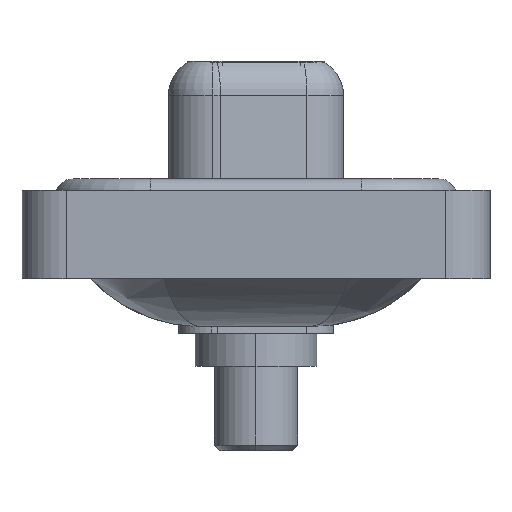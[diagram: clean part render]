
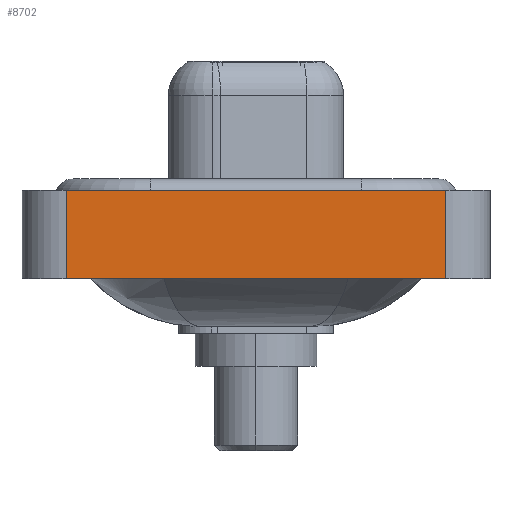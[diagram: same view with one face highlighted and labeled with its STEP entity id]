
A CAD part, left-side view. The second image highlights one B-rep face of the part: STEP entity #8702.
In plain terms, the highlighted planar face has unit normal (-1, 0, 0).
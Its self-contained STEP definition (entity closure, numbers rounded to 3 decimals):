
#165 = LINE ( 'NONE', #6627, #10528 ) ;
#203 = VECTOR ( 'NONE', #7106, 1000. ) ;
#679 = EDGE_CURVE ( 'NONE', #3708, #6044, #12628, .T. ) ;
#739 = VERTEX_POINT ( 'NONE', #1857 ) ;
#1495 = CARTESIAN_POINT ( 'NONE',  ( -7.3, 8.55, -3.6 ) ) ;
#1734 = ORIENTED_EDGE ( 'NONE', *, *, #12580, .T. ) ;
#1857 = CARTESIAN_POINT ( 'NONE',  ( -7.3, -8.55, -3.6 ) ) ;
#2555 = DIRECTION ( 'NONE',  ( 0., 0., 1. ) ) ;
#3118 = LINE ( 'NONE', #12574, #203 ) ;
#3282 = VECTOR ( 'NONE', #2555, 1000. ) ;
#3708 = VERTEX_POINT ( 'NONE', #15925 ) ;
#3989 = VECTOR ( 'NONE', #4555, 1000. ) ;
#4277 = DIRECTION ( 'NONE',  ( 0., -1., 0. ) ) ;
#4278 = CARTESIAN_POINT ( 'NONE',  ( -7.3, -8.55, 0.4 ) ) ;
#4555 = DIRECTION ( 'NONE',  ( 0., -1., 0. ) ) ;
#6044 = VERTEX_POINT ( 'NONE', #4278 ) ;
#6154 = DIRECTION ( 'NONE',  ( 0., 0., 1. ) ) ;
#6627 = CARTESIAN_POINT ( 'NONE',  ( -7.3, -8.55, -3.6 ) ) ;
#6684 = EDGE_LOOP ( 'NONE', ( #14309, #14378, #8694, #1734 ) ) ;
#7106 = DIRECTION ( 'NONE',  ( 0., 0., 1. ) ) ;
#8246 = EDGE_CURVE ( 'NONE', #739, #6044, #3118, .T. ) ;
#8694 = ORIENTED_EDGE ( 'NONE', *, *, #9217, .F. ) ;
#8702 = ADVANCED_FACE ( 'NONE', ( #9980 ), #11199, .T. ) ;
#9217 = EDGE_CURVE ( 'NONE', #12117, #3708, #14473, .T. ) ;
#9980 = FACE_OUTER_BOUND ( 'NONE', #6684, .T. ) ;
#10528 = VECTOR ( 'NONE', #4277, 1000. ) ;
#11199 = PLANE ( 'NONE',  #15180 ) ;
#12117 = VERTEX_POINT ( 'NONE', #1495 ) ;
#12506 = CARTESIAN_POINT ( 'NONE',  ( -7.3, -8.55, -3.6 ) ) ;
#12574 = CARTESIAN_POINT ( 'NONE',  ( -7.3, -8.55, -3.6 ) ) ;
#12580 = EDGE_CURVE ( 'NONE', #12117, #739, #165, .T. ) ;
#12628 = LINE ( 'NONE', #15325, #3989 ) ;
#12759 = DIRECTION ( 'NONE',  ( -1., 0., 0. ) ) ;
#14309 = ORIENTED_EDGE ( 'NONE', *, *, #8246, .T. ) ;
#14378 = ORIENTED_EDGE ( 'NONE', *, *, #679, .F. ) ;
#14473 = LINE ( 'NONE', #16816, #3282 ) ;
#15180 = AXIS2_PLACEMENT_3D ( 'NONE', #12506, #12759, #6154 ) ;
#15325 = CARTESIAN_POINT ( 'NONE',  ( -7.3, -8.55, 0.4 ) ) ;
#15925 = CARTESIAN_POINT ( 'NONE',  ( -7.3, 8.55, 0.4 ) ) ;
#16816 = CARTESIAN_POINT ( 'NONE',  ( -7.3, 8.55, -3.6 ) ) ;
